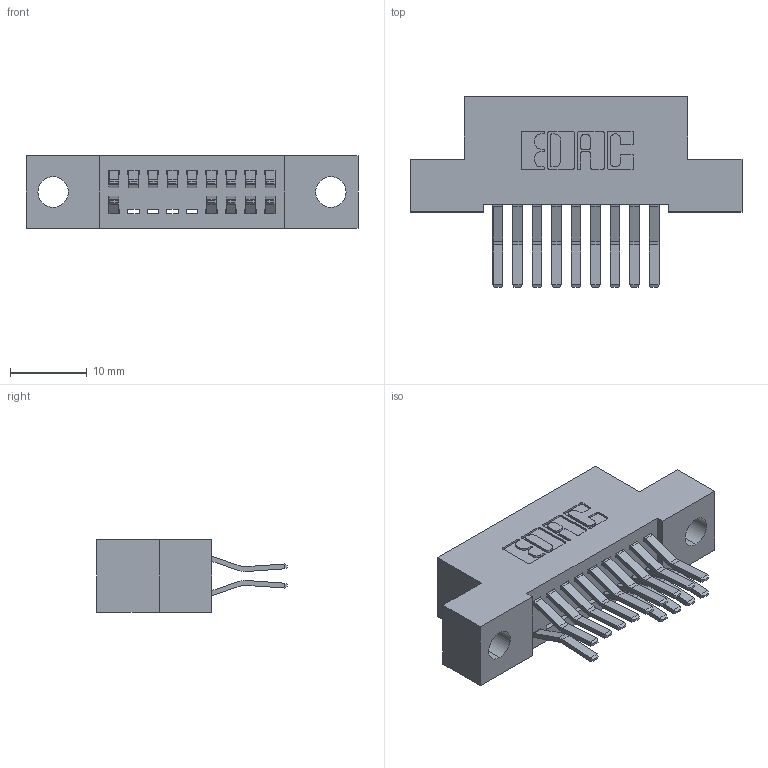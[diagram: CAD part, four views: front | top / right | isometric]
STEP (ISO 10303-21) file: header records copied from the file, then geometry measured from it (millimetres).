
FILE_DESCRIPTION (( 'STEP AP203' ), '1' );
FILE_NAME ('392-018-560-204.STEP', '2018-08-15T05:02:57', ( '' ), ( '' ), 'SwSTEP 2.0', 'SolidWorks 2016', '' );
FILE_SCHEMA (( 'CONFIG_CONTROL_DESIGN' ));
Length unit declared in the file: inch
Products named in the file (3): 342 Part_.156 TH; 345-292-001_560 Tail; 392-018-560-204
Assembly tree (15 placements, depth 2):
  392-018-560-204
    342 Part_.156 TH
    345-292-001_560 Tail  x14
Bounding box: 43.18 x 24.78 x 9.4 mm (x, y, z)
Volume: 3692.4 mm3; surface area: 5042.8 mm2
Topology: 15 solids, 15 shells, 890 faces, 2637 edges, 1738 vertices
Faces by surface type: plane 594, cylinder 296
Entity records: 9889 total; most frequent: CARTESIAN_POINT 1694, ORIENTED_EDGE 1634, DIRECTION 1505, EDGE_CURVE 817, VECTOR 685, LINE 685, VERTEX_POINT 542, AXIS2_PLACEMENT_3D 410
